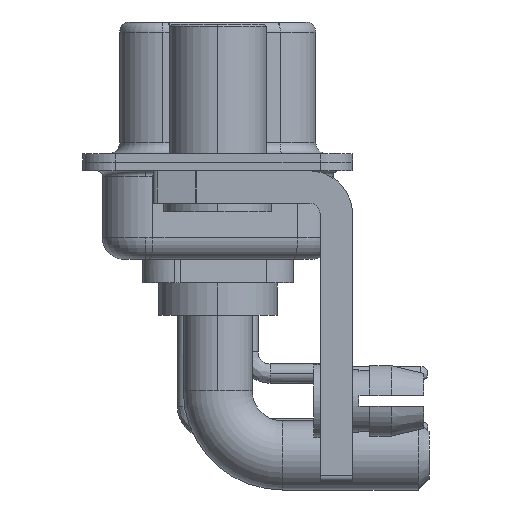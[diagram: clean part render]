
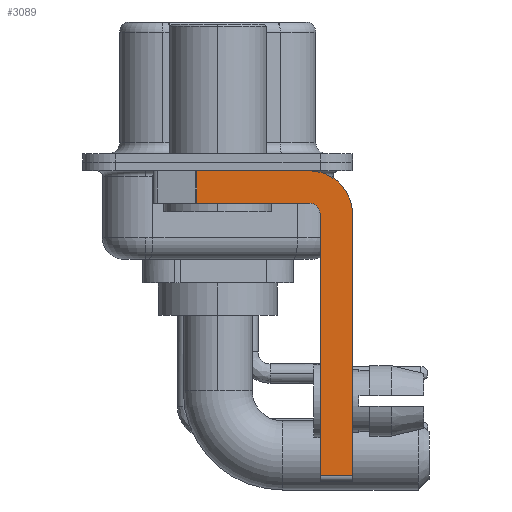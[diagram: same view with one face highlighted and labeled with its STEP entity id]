
A CAD part, left-side view. The second image highlights one B-rep face of the part: STEP entity #3089.
In plain terms, the highlighted planar face has unit normal (-1, 0, 0).
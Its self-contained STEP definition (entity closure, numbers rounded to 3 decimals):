
#280 = DIRECTION ( 'NONE',  ( -1., 0., 0. ) ) ;
#973 = PLANE ( 'NONE',  #17001 ) ;
#974 = VERTEX_POINT ( 'NONE', #13282 ) ;
#1032 = VERTEX_POINT ( 'NONE', #17609 ) ;
#2264 = DIRECTION ( 'NONE',  ( 0., -1., 0. ) ) ;
#3089 = ADVANCED_FACE ( 'NONE', ( #25958 ), #973, .F. ) ;
#3221 = DIRECTION ( 'NONE',  ( 1., 0., 0. ) ) ;
#3594 = ORIENTED_EDGE ( 'NONE', *, *, #29492, .T. ) ;
#4392 = ORIENTED_EDGE ( 'NONE', *, *, #6533, .F. ) ;
#4466 = CARTESIAN_POINT ( 'NONE',  ( -2.9, -6.25, -2.4 ) ) ;
#4591 = VERTEX_POINT ( 'NONE', #15324 ) ;
#4762 = ORIENTED_EDGE ( 'NONE', *, *, #9753, .F. ) ;
#5224 = EDGE_CURVE ( 'NONE', #30100, #4591, #9394, .T. ) ;
#5914 = LINE ( 'NONE', #22942, #27087 ) ;
#6166 = DIRECTION ( 'NONE',  ( 1., 0., 0. ) ) ;
#6352 = CIRCLE ( 'NONE', #15639, 2. ) ;
#6533 = EDGE_CURVE ( 'NONE', #974, #21127, #11755, .T. ) ;
#6547 = CARTESIAN_POINT ( 'NONE',  ( -2.9, 0.978, -1.9 ) ) ;
#6746 = VERTEX_POINT ( 'NONE', #8322 ) ;
#7034 = EDGE_LOOP ( 'NONE', ( #9414, #11340, #13797, #20984, #24548, #3594, #4392, #4762 ) ) ;
#7206 = DIRECTION ( 'NONE',  ( 0., 0., -1. ) ) ;
#8274 = DIRECTION ( 'NONE',  ( 0., 0., -1. ) ) ;
#8322 = CARTESIAN_POINT ( 'NONE',  ( -2.9, -4.75, -2.4 ) ) ;
#9394 = LINE ( 'NONE', #19317, #21935 ) ;
#9414 = ORIENTED_EDGE ( 'NONE', *, *, #5224, .F. ) ;
#9496 = CARTESIAN_POINT ( 'NONE',  ( -2.9, -6.25, -14.55 ) ) ;
#9753 = EDGE_CURVE ( 'NONE', #4591, #974, #6352, .T. ) ;
#11340 = ORIENTED_EDGE ( 'NONE', *, *, #18853, .T. ) ;
#11755 = LINE ( 'NONE', #4466, #16805 ) ;
#11938 = CARTESIAN_POINT ( 'NONE',  ( -2.9, -4.75, -14.55 ) ) ;
#12747 = CARTESIAN_POINT ( 'NONE',  ( -2.9, -4.25, -2.4 ) ) ;
#13282 = CARTESIAN_POINT ( 'NONE',  ( -2.9, -6.25, -2.4 ) ) ;
#13627 = CARTESIAN_POINT ( 'NONE',  ( -2.9, 0.978, -0.4 ) ) ;
#13797 = ORIENTED_EDGE ( 'NONE', *, *, #29569, .F. ) ;
#13898 = DIRECTION ( 'NONE',  ( 0., 0., 1. ) ) ;
#14377 = CARTESIAN_POINT ( 'NONE',  ( -2.9, -4.75, -14.8 ) ) ;
#14480 = AXIS2_PLACEMENT_3D ( 'NONE', #12747, #280, #17618 ) ;
#15324 = CARTESIAN_POINT ( 'NONE',  ( -2.9, -4.25, -0.4 ) ) ;
#15450 = DIRECTION ( 'NONE',  ( 0., 1., 0. ) ) ;
#15639 = AXIS2_PLACEMENT_3D ( 'NONE', #18456, #3221, #28202 ) ;
#16805 = VECTOR ( 'NONE', #7206, 1000. ) ;
#17001 = AXIS2_PLACEMENT_3D ( 'NONE', #30518, #6166, #8274 ) ;
#17609 = CARTESIAN_POINT ( 'NONE',  ( -2.9, 0.978, -1.9 ) ) ;
#17618 = DIRECTION ( 'NONE',  ( 0., 0., 1. ) ) ;
#18456 = CARTESIAN_POINT ( 'NONE',  ( -2.9, -4.25, -2.4 ) ) ;
#18542 = LINE ( 'NONE', #30267, #19295 ) ;
#18853 = EDGE_CURVE ( 'NONE', #30100, #1032, #26327, .T. ) ;
#19295 = VECTOR ( 'NONE', #23099, 1000. ) ;
#19317 = CARTESIAN_POINT ( 'NONE',  ( -2.9, 3., -0.4 ) ) ;
#20569 = EDGE_CURVE ( 'NONE', #25490, #6746, #21230, .T. ) ;
#20984 = ORIENTED_EDGE ( 'NONE', *, *, #26820, .F. ) ;
#21127 = VERTEX_POINT ( 'NONE', #9496 ) ;
#21230 = LINE ( 'NONE', #14377, #31207 ) ;
#21935 = VECTOR ( 'NONE', #2264, 1000. ) ;
#22942 = CARTESIAN_POINT ( 'NONE',  ( -2.9, -4.25, -1.9 ) ) ;
#23099 = DIRECTION ( 'NONE',  ( 0., -1., 0. ) ) ;
#24548 = ORIENTED_EDGE ( 'NONE', *, *, #20569, .F. ) ;
#25490 = VERTEX_POINT ( 'NONE', #11938 ) ;
#25769 = CARTESIAN_POINT ( 'NONE',  ( -2.9, -4.25, -1.9 ) ) ;
#25958 = FACE_OUTER_BOUND ( 'NONE', #7034, .T. ) ;
#26327 = LINE ( 'NONE', #6547, #26343 ) ;
#26343 = VECTOR ( 'NONE', #31046, 1000. ) ;
#26820 = EDGE_CURVE ( 'NONE', #6746, #31779, #26931, .T. ) ;
#26931 = CIRCLE ( 'NONE', #14480, 0.5 ) ;
#27087 = VECTOR ( 'NONE', #15450, 1000. ) ;
#28202 = DIRECTION ( 'NONE',  ( 0., 0., -1. ) ) ;
#29492 = EDGE_CURVE ( 'NONE', #25490, #21127, #18542, .T. ) ;
#29569 = EDGE_CURVE ( 'NONE', #31779, #1032, #5914, .T. ) ;
#30100 = VERTEX_POINT ( 'NONE', #13627 ) ;
#30267 = CARTESIAN_POINT ( 'NONE',  ( -2.9, -4.25, -14.55 ) ) ;
#30518 = CARTESIAN_POINT ( 'NONE',  ( -2.9, -4.25, -2.4 ) ) ;
#31046 = DIRECTION ( 'NONE',  ( 0., 0., -1. ) ) ;
#31207 = VECTOR ( 'NONE', #13898, 1000. ) ;
#31779 = VERTEX_POINT ( 'NONE', #25769 ) ;
